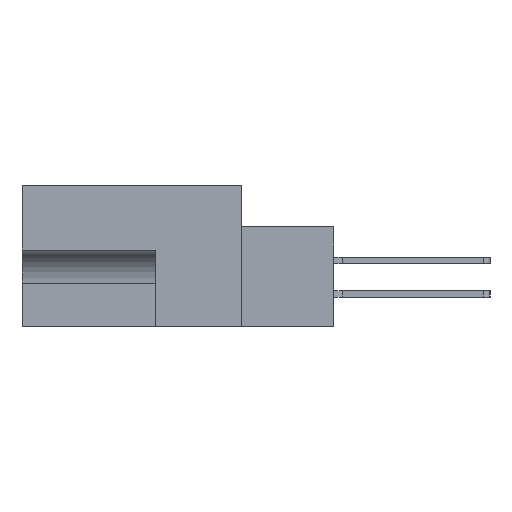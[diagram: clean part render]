
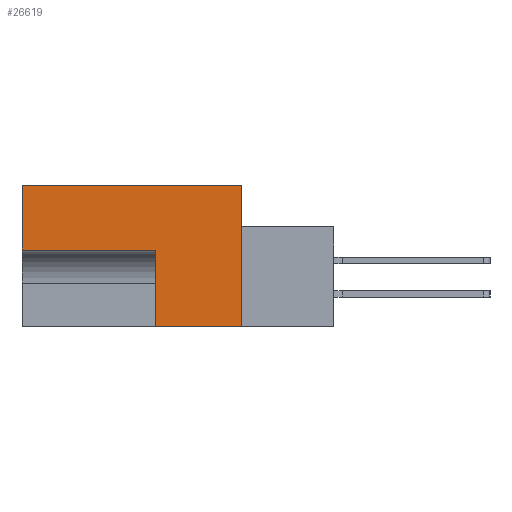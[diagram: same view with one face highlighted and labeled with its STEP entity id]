
A CAD part, left-side view. The second image highlights one B-rep face of the part: STEP entity #26619.
In plain terms, the highlighted planar face has unit normal (-1, 0, 0).
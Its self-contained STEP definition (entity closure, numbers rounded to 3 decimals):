
#1315 = EDGE_CURVE ( 'NONE', #8035, #34366, #37093, .T. ) ;
#1407 = VECTOR ( 'NONE', #32457, 1000. ) ;
#1662 = EDGE_CURVE ( 'NONE', #11343, #5146, #32644, .T. ) ;
#3081 = LINE ( 'NONE', #17820, #5532 ) ;
#3175 = LINE ( 'NONE', #4118, #31234 ) ;
#3718 = VECTOR ( 'NONE', #31377, 1000. ) ;
#4118 = CARTESIAN_POINT ( 'NONE',  ( 0., -8.814, -13.487 ) ) ;
#5146 = VERTEX_POINT ( 'NONE', #15067 ) ;
#5424 = ORIENTED_EDGE ( 'NONE', *, *, #1315, .F. ) ;
#5532 = VECTOR ( 'NONE', #31167, 1000. ) ;
#8035 = VERTEX_POINT ( 'NONE', #39402 ) ;
#8053 = AXIS2_PLACEMENT_3D ( 'NONE', #33123, #26764, #20727 ) ;
#10123 = EDGE_CURVE ( 'NONE', #34366, #11343, #3081, .T. ) ;
#10289 = CARTESIAN_POINT ( 'NONE',  ( 0., 0., 0. ) ) ;
#11343 = VERTEX_POINT ( 'NONE', #13287 ) ;
#12364 = CARTESIAN_POINT ( 'NONE',  ( 0., 20.955, -6.172 ) ) ;
#13287 = CARTESIAN_POINT ( 'NONE',  ( 0., 20.955, 0. ) ) ;
#13842 = CARTESIAN_POINT ( 'NONE',  ( 0., 8.255, -6.172 ) ) ;
#14641 = PLANE ( 'NONE',  #8053 ) ;
#15009 = LINE ( 'NONE', #31782, #3718 ) ;
#15067 = CARTESIAN_POINT ( 'NONE',  ( 0., 0., 0. ) ) ;
#16461 = CARTESIAN_POINT ( 'NONE',  ( 0., 0., -13.487 ) ) ;
#17820 = CARTESIAN_POINT ( 'NONE',  ( 0., 20.955, -13.487 ) ) ;
#17878 = VECTOR ( 'NONE', #20166, 1000. ) ;
#19450 = ORIENTED_EDGE ( 'NONE', *, *, #20268, .F. ) ;
#19835 = VECTOR ( 'NONE', #34736, 1000. ) ;
#20166 = DIRECTION ( 'NONE',  ( 0., 1., 0. ) ) ;
#20268 = EDGE_CURVE ( 'NONE', #23170, #36267, #3175, .T. ) ;
#20727 = DIRECTION ( 'NONE',  ( 0., 0., -1. ) ) ;
#21425 = FACE_OUTER_BOUND ( 'NONE', #36865, .T. ) ;
#22475 = ORIENTED_EDGE ( 'NONE', *, *, #27455, .F. ) ;
#23170 = VERTEX_POINT ( 'NONE', #16461 ) ;
#23373 = DIRECTION ( 'NONE',  ( 0., 1., 0. ) ) ;
#24250 = ORIENTED_EDGE ( 'NONE', *, *, #1662, .F. ) ;
#25793 = CARTESIAN_POINT ( 'NONE',  ( 0., 8.255, -13.487 ) ) ;
#26619 = ADVANCED_FACE ( 'NONE', ( #21425 ), #14641, .F. ) ;
#26764 = DIRECTION ( 'NONE',  ( 1., 0., 0. ) ) ;
#27455 = EDGE_CURVE ( 'NONE', #36267, #8035, #15009, .T. ) ;
#27883 = ORIENTED_EDGE ( 'NONE', *, *, #10123, .F. ) ;
#29922 = ORIENTED_EDGE ( 'NONE', *, *, #40777, .F. ) ;
#31167 = DIRECTION ( 'NONE',  ( 0., 0., 1. ) ) ;
#31234 = VECTOR ( 'NONE', #23373, 1000. ) ;
#31377 = DIRECTION ( 'NONE',  ( 0., 0., 1. ) ) ;
#31782 = CARTESIAN_POINT ( 'NONE',  ( 0., 8.255, -13.487 ) ) ;
#32457 = DIRECTION ( 'NONE',  ( 0., 0., -1. ) ) ;
#32644 = LINE ( 'NONE', #37914, #19835 ) ;
#32895 = LINE ( 'NONE', #10289, #1407 ) ;
#33123 = CARTESIAN_POINT ( 'NONE',  ( 0., 0., 0. ) ) ;
#34366 = VERTEX_POINT ( 'NONE', #12364 ) ;
#34736 = DIRECTION ( 'NONE',  ( 0., -1., 0. ) ) ;
#36267 = VERTEX_POINT ( 'NONE', #25793 ) ;
#36865 = EDGE_LOOP ( 'NONE', ( #19450, #29922, #24250, #27883, #5424, #22475 ) ) ;
#37093 = LINE ( 'NONE', #13842, #17878 ) ;
#37914 = CARTESIAN_POINT ( 'NONE',  ( 0., 11.506, 0. ) ) ;
#39402 = CARTESIAN_POINT ( 'NONE',  ( 0., 8.255, -6.172 ) ) ;
#40777 = EDGE_CURVE ( 'NONE', #5146, #23170, #32895, .T. ) ;
